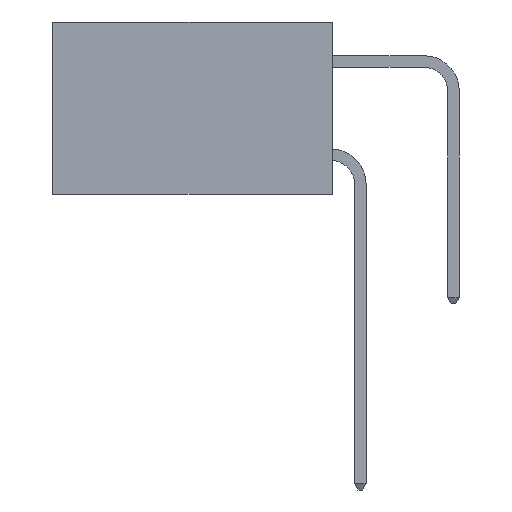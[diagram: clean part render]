
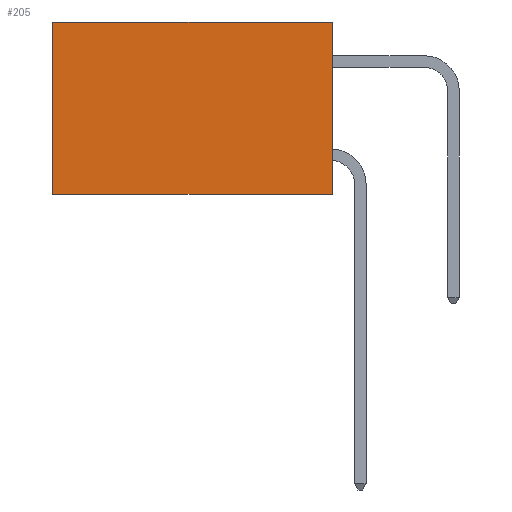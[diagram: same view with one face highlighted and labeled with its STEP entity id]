
A CAD part, left-side view. The second image highlights one B-rep face of the part: STEP entity #205.
In plain terms, the highlighted planar face has unit normal (-1, 0, 0).
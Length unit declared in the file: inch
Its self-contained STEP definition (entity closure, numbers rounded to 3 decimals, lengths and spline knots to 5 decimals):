
#28 = EDGE_CURVE ( 'NONE', #2704, #758, #1566, .T. ) ;
#205 = ADVANCED_FACE ( 'NONE', ( #8948 ), #5437, .F. ) ;
#758 = VERTEX_POINT ( 'NONE', #5613 ) ;
#1266 = ORIENTED_EDGE ( 'NONE', *, *, #28, .T. ) ;
#1275 = ORIENTED_EDGE ( 'NONE', *, *, #3038, .F. ) ;
#1299 = ORIENTED_EDGE ( 'NONE', *, *, #3582, .F. ) ;
#1307 = ORIENTED_EDGE ( 'NONE', *, *, #7387, .T. ) ;
#1566 = LINE ( 'NONE', #5292, #3538 ) ;
#1591 = VECTOR ( 'NONE', #9350, 39.37008 ) ;
#1818 = EDGE_LOOP ( 'NONE', ( #1266, #1275, #1299, #1307 ) ) ;
#2004 = VECTOR ( 'NONE', #3090, 39.37008 ) ;
#2704 = VERTEX_POINT ( 'NONE', #4607 ) ;
#3038 = EDGE_CURVE ( 'NONE', #8984, #758, #8152, .T. ) ;
#3090 = DIRECTION ( 'NONE',  ( 0., 1., 0. ) ) ;
#3212 = CARTESIAN_POINT ( 'NONE',  ( 0.2615, 0., -0.37 ) ) ;
#3538 = VECTOR ( 'NONE', #5548, 39.37008 ) ;
#3582 = EDGE_CURVE ( 'NONE', #4887, #8984, #9381, .T. ) ;
#4038 = CARTESIAN_POINT ( 'NONE',  ( 0.2615, 0., 0. ) ) ;
#4200 = DIRECTION ( 'NONE',  ( 0., 0., -1. ) ) ;
#4607 = CARTESIAN_POINT ( 'NONE',  ( 0.2615, 0.6, 0. ) ) ;
#4887 = VERTEX_POINT ( 'NONE', #8825 ) ;
#5117 = LINE ( 'NONE', #4038, #8244 ) ;
#5292 = CARTESIAN_POINT ( 'NONE',  ( 0.2615, 0.6, -0.37 ) ) ;
#5437 = PLANE ( 'NONE',  #5575 ) ;
#5512 = DIRECTION ( 'NONE',  ( 1., 0., 0. ) ) ;
#5548 = DIRECTION ( 'NONE',  ( 0., 0., -1. ) ) ;
#5575 = AXIS2_PLACEMENT_3D ( 'NONE', #8263, #5512, #4200 ) ;
#5613 = CARTESIAN_POINT ( 'NONE',  ( 0.2615, 0.6, -0.37 ) ) ;
#6435 = DIRECTION ( 'NONE',  ( 0., 1., 0. ) ) ;
#7387 = EDGE_CURVE ( 'NONE', #4887, #2704, #5117, .T. ) ;
#7511 = CARTESIAN_POINT ( 'NONE',  ( 0.2615, 0., -0.37 ) ) ;
#8152 = LINE ( 'NONE', #3212, #2004 ) ;
#8244 = VECTOR ( 'NONE', #6435, 39.37008 ) ;
#8263 = CARTESIAN_POINT ( 'NONE',  ( 0.2615, 0., -0.37 ) ) ;
#8825 = CARTESIAN_POINT ( 'NONE',  ( 0.2615, 0., 0. ) ) ;
#8948 = FACE_OUTER_BOUND ( 'NONE', #1818, .T. ) ;
#8984 = VERTEX_POINT ( 'NONE', #7511 ) ;
#9350 = DIRECTION ( 'NONE',  ( 0., 0., -1. ) ) ;
#9381 = LINE ( 'NONE', #9966, #1591 ) ;
#9966 = CARTESIAN_POINT ( 'NONE',  ( 0.2615, 0., -0.37 ) ) ;
